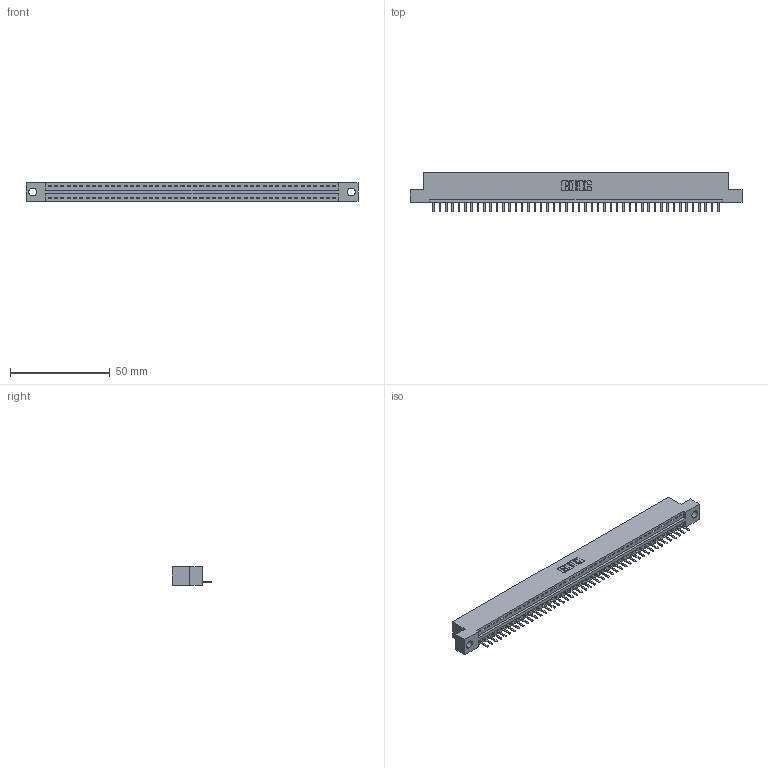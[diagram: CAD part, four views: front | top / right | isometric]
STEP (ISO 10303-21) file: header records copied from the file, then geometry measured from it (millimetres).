
FILE_DESCRIPTION (( 'STEP AP203' ), '1' );
FILE_NAME ('346-046-520-104.STEP', '2022-05-09T19:33:38', ( '' ), ( '' ), 'SwSTEP 2.0', 'SolidWorks 2020', '' );
FILE_SCHEMA (( 'CONFIG_CONTROL_DESIGN' ));
Length unit declared in the file: inch
Products named in the file (3): 346 Part_Flush Mounting Lugs - 0.156 Dia-TH; 346-046-520-104; 345-292-001_345-293-120
Assembly tree (47 placements, depth 2):
  346-046-520-104
    346 Part_Flush Mounting Lugs - 0.156 Dia-TH
    345-292-001_345-293-120  x46
Bounding box: 166.62 x 20.02 x 9.4 mm (x, y, z)
Volume: 15738.9 mm3; surface area: 19110.3 mm2
Topology: 47 solids, 47 shells, 2988 faces, 8829 edges, 5762 vertices
Faces by surface type: plane 2022, cylinder 966
Entity records: 28543 total; most frequent: CARTESIAN_POINT 4912, ORIENTED_EDGE 4878, DIRECTION 4315, EDGE_CURVE 2439, LINE 2119, VECTOR 2119, VERTEX_POINT 1622, AXIS2_PLACEMENT_3D 1098
